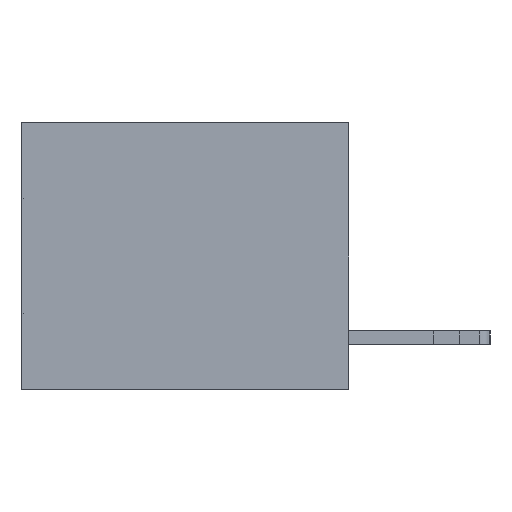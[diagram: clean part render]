
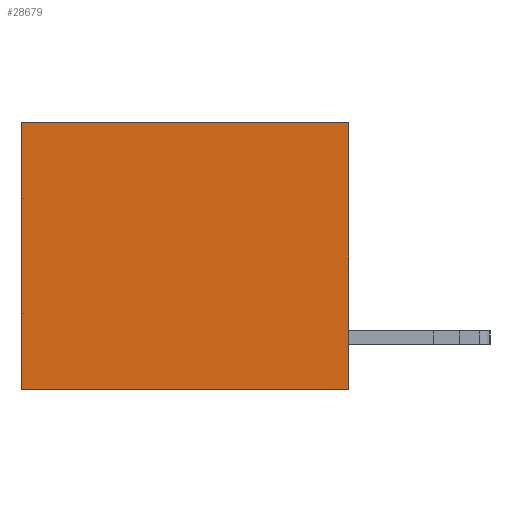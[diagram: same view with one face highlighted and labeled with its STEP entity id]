
A CAD part, left-side view. The second image highlights one B-rep face of the part: STEP entity #28679.
In plain terms, the highlighted planar face has unit normal (-1, 0, 0).
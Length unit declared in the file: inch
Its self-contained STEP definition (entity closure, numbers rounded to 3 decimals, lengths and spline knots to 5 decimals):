
#873 = FACE_OUTER_BOUND ( 'NONE', #15936, .T. ) ;
#1263 = CARTESIAN_POINT ( 'NONE',  ( 0.3165, 0.6, 0. ) ) ;
#1613 = DIRECTION ( 'NONE',  ( 0., 0., -1. ) ) ;
#1688 = LINE ( 'NONE', #12791, #20185 ) ;
#2147 = VERTEX_POINT ( 'NONE', #20331 ) ;
#2489 = DIRECTION ( 'NONE',  ( 0., 1., 0. ) ) ;
#4160 = VERTEX_POINT ( 'NONE', #1263 ) ;
#5437 = EDGE_CURVE ( 'NONE', #17359, #4160, #27667, .T. ) ;
#5796 = VECTOR ( 'NONE', #12358, 39.37008 ) ;
#6818 = CARTESIAN_POINT ( 'NONE',  ( 0.3165, 0., 0. ) ) ;
#7580 = CARTESIAN_POINT ( 'NONE',  ( 0.3165, 0., -0.49 ) ) ;
#7649 = CARTESIAN_POINT ( 'NONE',  ( 0.3165, 0., -0.49 ) ) ;
#9955 = CARTESIAN_POINT ( 'NONE',  ( 0.3165, 0., -0.49 ) ) ;
#12277 = CARTESIAN_POINT ( 'NONE',  ( 0.3165, 0., 0. ) ) ;
#12358 = DIRECTION ( 'NONE',  ( 0., 1., 0. ) ) ;
#12791 = CARTESIAN_POINT ( 'NONE',  ( 0.3165, 0.6, -0.49 ) ) ;
#13531 = VECTOR ( 'NONE', #2489, 39.37008 ) ;
#14367 = PLANE ( 'NONE',  #16339 ) ;
#14725 = EDGE_CURVE ( 'NONE', #31266, #2147, #16441, .T. ) ;
#15926 = VECTOR ( 'NONE', #17492, 39.37008 ) ;
#15936 = EDGE_LOOP ( 'NONE', ( #29222, #27049, #17692, #32401 ) ) ;
#16339 = AXIS2_PLACEMENT_3D ( 'NONE', #16805, #31727, #1613 ) ;
#16441 = LINE ( 'NONE', #9955, #5796 ) ;
#16805 = CARTESIAN_POINT ( 'NONE',  ( 0.3165, 0., -0.49 ) ) ;
#17359 = VERTEX_POINT ( 'NONE', #6818 ) ;
#17492 = DIRECTION ( 'NONE',  ( 0., 0., -1. ) ) ;
#17692 = ORIENTED_EDGE ( 'NONE', *, *, #19134, .F. ) ;
#19134 = EDGE_CURVE ( 'NONE', #17359, #31266, #26150, .T. ) ;
#19863 = EDGE_CURVE ( 'NONE', #4160, #2147, #1688, .T. ) ;
#20185 = VECTOR ( 'NONE', #22876, 39.37008 ) ;
#20331 = CARTESIAN_POINT ( 'NONE',  ( 0.3165, 0.6, -0.49 ) ) ;
#22876 = DIRECTION ( 'NONE',  ( 0., 0., -1. ) ) ;
#26150 = LINE ( 'NONE', #7580, #15926 ) ;
#27049 = ORIENTED_EDGE ( 'NONE', *, *, #14725, .F. ) ;
#27667 = LINE ( 'NONE', #12277, #13531 ) ;
#28679 = ADVANCED_FACE ( 'NONE', ( #873 ), #14367, .F. ) ;
#29222 = ORIENTED_EDGE ( 'NONE', *, *, #19863, .T. ) ;
#31266 = VERTEX_POINT ( 'NONE', #7649 ) ;
#31727 = DIRECTION ( 'NONE',  ( 1., 0., 0. ) ) ;
#32401 = ORIENTED_EDGE ( 'NONE', *, *, #5437, .T. ) ;
